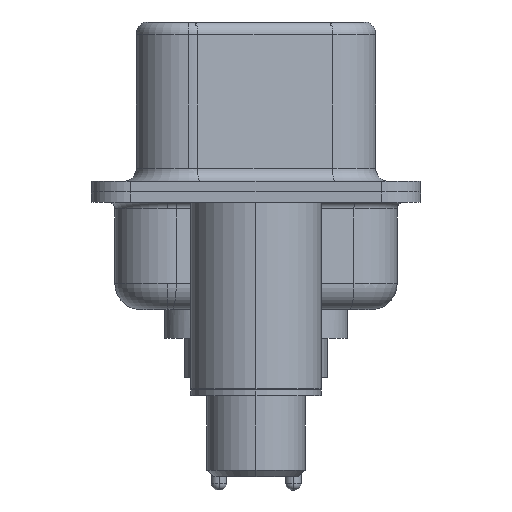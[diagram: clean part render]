
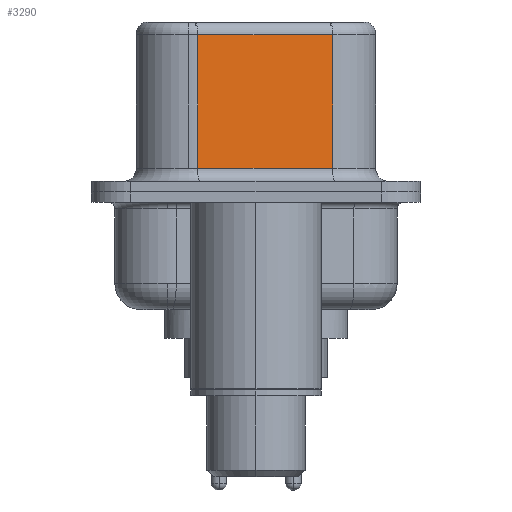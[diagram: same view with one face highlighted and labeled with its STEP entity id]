
A CAD part, left-side view. The second image highlights one B-rep face of the part: STEP entity #3290.
In plain terms, the highlighted planar face has unit normal (-0.985, -0.174, 0).
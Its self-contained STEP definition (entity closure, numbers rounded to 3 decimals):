
#24 = VERTEX_POINT ( 'NONE', #2324 ) ;
#276 = ORIENTED_EDGE ( 'NONE', *, *, #17526, .T. ) ;
#288 = DIRECTION ( 'NONE',  ( 0., 0., -1. ) ) ;
#2324 = CARTESIAN_POINT ( 'NONE',  ( 4.58, -2.927, 0.9 ) ) ;
#3290 = ADVANCED_FACE ( 'NONE', ( #20340 ), #4748, .F. ) ;
#4748 = PLANE ( 'NONE',  #20068 ) ;
#5097 = ORIENTED_EDGE ( 'NONE', *, *, #15126, .F. ) ;
#6732 = EDGE_CURVE ( 'NONE', #9380, #8320, #12566, .T. ) ;
#7024 = LINE ( 'NONE', #7213, #15528 ) ;
#7213 = CARTESIAN_POINT ( 'NONE',  ( 4.58, -2.927, 6.52 ) ) ;
#7624 = DIRECTION ( 'NONE',  ( 0.985, 0.174, 0. ) ) ;
#7677 = DIRECTION ( 'NONE',  ( -0.174, 0.985, 0. ) ) ;
#8320 = VERTEX_POINT ( 'NONE', #21273 ) ;
#8464 = CARTESIAN_POINT ( 'NONE',  ( 4.58, -2.927, 0.9 ) ) ;
#8933 = EDGE_LOOP ( 'NONE', ( #5097, #20531, #276, #18703 ) ) ;
#9380 = VERTEX_POINT ( 'NONE', #13871 ) ;
#10263 = CARTESIAN_POINT ( 'NONE',  ( 3.67, 2.233, 6.52 ) ) ;
#11802 = VECTOR ( 'NONE', #11945, 1000. ) ;
#11945 = DIRECTION ( 'NONE',  ( 0., 0., -1. ) ) ;
#12108 = VECTOR ( 'NONE', #15256, 1000. ) ;
#12566 = LINE ( 'NONE', #14425, #15974 ) ;
#13871 = CARTESIAN_POINT ( 'NONE',  ( 4.58, -2.927, 6.02 ) ) ;
#14272 = DIRECTION ( 'NONE',  ( -0.174, 0.985, 0. ) ) ;
#14425 = CARTESIAN_POINT ( 'NONE',  ( 4.58, -2.927, 6.02 ) ) ;
#15126 = EDGE_CURVE ( 'NONE', #9380, #24, #7024, .T. ) ;
#15256 = DIRECTION ( 'NONE',  ( 0.174, -0.985, 0. ) ) ;
#15528 = VECTOR ( 'NONE', #288, 1000. ) ;
#15974 = VECTOR ( 'NONE', #14272, 1000. ) ;
#16224 = EDGE_CURVE ( 'NONE', #18471, #24, #16573, .T. ) ;
#16253 = LINE ( 'NONE', #10263, #11802 ) ;
#16573 = LINE ( 'NONE', #8464, #12108 ) ;
#17526 = EDGE_CURVE ( 'NONE', #8320, #18471, #16253, .T. ) ;
#17556 = CARTESIAN_POINT ( 'NONE',  ( 3.67, 2.233, 0.9 ) ) ;
#18471 = VERTEX_POINT ( 'NONE', #17556 ) ;
#18703 = ORIENTED_EDGE ( 'NONE', *, *, #16224, .T. ) ;
#19093 = CARTESIAN_POINT ( 'NONE',  ( 4.58, -2.927, 6.52 ) ) ;
#20068 = AXIS2_PLACEMENT_3D ( 'NONE', #19093, #7624, #7677 ) ;
#20340 = FACE_OUTER_BOUND ( 'NONE', #8933, .T. ) ;
#20531 = ORIENTED_EDGE ( 'NONE', *, *, #6732, .T. ) ;
#21273 = CARTESIAN_POINT ( 'NONE',  ( 3.67, 2.233, 6.02 ) ) ;
